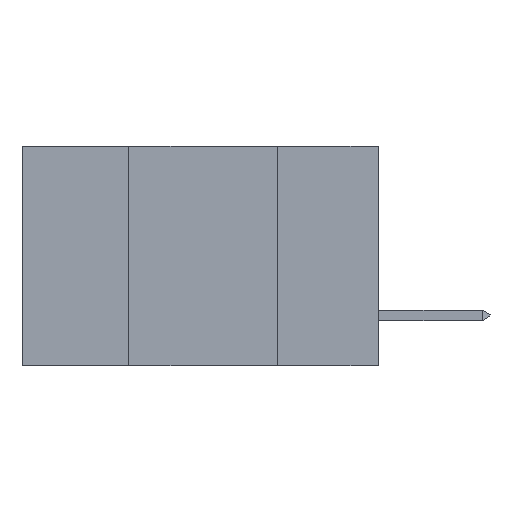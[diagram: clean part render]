
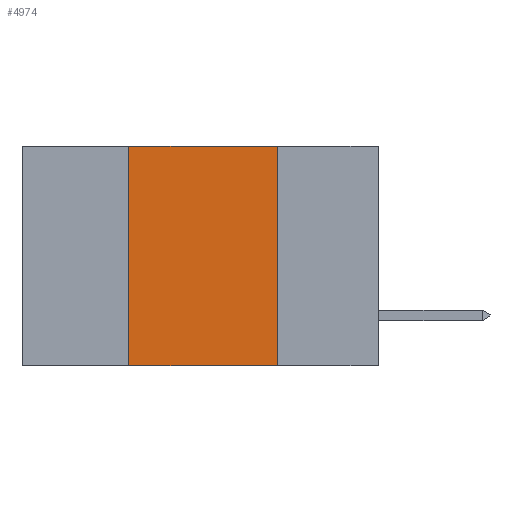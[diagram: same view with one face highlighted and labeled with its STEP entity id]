
A CAD part, left-side view. The second image highlights one B-rep face of the part: STEP entity #4974.
In plain terms, the highlighted planar face has unit normal (-1, 0, 0).
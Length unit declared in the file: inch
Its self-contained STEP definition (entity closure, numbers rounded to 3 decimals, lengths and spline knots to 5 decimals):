
#143 = VECTOR ( 'NONE', #13820, 39.37008 ) ;
#227 = EDGE_CURVE ( 'NONE', #4070, #11540, #445, .T. ) ;
#445 = LINE ( 'NONE', #10763, #6749 ) ;
#1224 = FACE_OUTER_BOUND ( 'NONE', #3802, .T. ) ;
#1285 = CARTESIAN_POINT ( 'NONE',  ( 0., 0.42, -0.37 ) ) ;
#1436 = EDGE_CURVE ( 'NONE', #11540, #12317, #7944, .T. ) ;
#3243 = AXIS2_PLACEMENT_3D ( 'NONE', #9977, #7388, #4977 ) ;
#3629 = LINE ( 'NONE', #8709, #143 ) ;
#3802 = EDGE_LOOP ( 'NONE', ( #9875, #9146, #6564, #7541 ) ) ;
#4070 = VERTEX_POINT ( 'NONE', #8532 ) ;
#4945 = LINE ( 'NONE', #10100, #6835 ) ;
#4974 = ADVANCED_FACE ( 'NONE', ( #1224 ), #6056, .F. ) ;
#4977 = DIRECTION ( 'NONE',  ( 0., 0., -1. ) ) ;
#5740 = CARTESIAN_POINT ( 'NONE',  ( 0., 0.17, 0. ) ) ;
#6056 = PLANE ( 'NONE',  #3243 ) ;
#6564 = ORIENTED_EDGE ( 'NONE', *, *, #12629, .F. ) ;
#6749 = VECTOR ( 'NONE', #9511, 39.37008 ) ;
#6835 = VECTOR ( 'NONE', #16408, 39.37008 ) ;
#7388 = DIRECTION ( 'NONE',  ( 1., 0., 0. ) ) ;
#7541 = ORIENTED_EDGE ( 'NONE', *, *, #14265, .T. ) ;
#7944 = LINE ( 'NONE', #15477, #10342 ) ;
#8532 = CARTESIAN_POINT ( 'NONE',  ( 0., 0.42, 0. ) ) ;
#8709 = CARTESIAN_POINT ( 'NONE',  ( 0., 0.42, -0.37 ) ) ;
#9146 = ORIENTED_EDGE ( 'NONE', *, *, #227, .F. ) ;
#9511 = DIRECTION ( 'NONE',  ( 0., -1., 0. ) ) ;
#9875 = ORIENTED_EDGE ( 'NONE', *, *, #1436, .F. ) ;
#9977 = CARTESIAN_POINT ( 'NONE',  ( 0., 0.6, 0. ) ) ;
#10100 = CARTESIAN_POINT ( 'NONE',  ( 0., 0.6, -0.37 ) ) ;
#10342 = VECTOR ( 'NONE', #15567, 39.37008 ) ;
#10450 = VERTEX_POINT ( 'NONE', #1285 ) ;
#10763 = CARTESIAN_POINT ( 'NONE',  ( 0., 0.6, 0. ) ) ;
#11540 = VERTEX_POINT ( 'NONE', #5740 ) ;
#12317 = VERTEX_POINT ( 'NONE', #14422 ) ;
#12629 = EDGE_CURVE ( 'NONE', #10450, #4070, #3629, .T. ) ;
#13820 = DIRECTION ( 'NONE',  ( 0., 0., 1. ) ) ;
#14265 = EDGE_CURVE ( 'NONE', #10450, #12317, #4945, .T. ) ;
#14422 = CARTESIAN_POINT ( 'NONE',  ( 0., 0.17, -0.37 ) ) ;
#15477 = CARTESIAN_POINT ( 'NONE',  ( 0., 0.17, -0.37 ) ) ;
#15567 = DIRECTION ( 'NONE',  ( 0., 0., -1. ) ) ;
#16408 = DIRECTION ( 'NONE',  ( 0., -1., 0. ) ) ;
